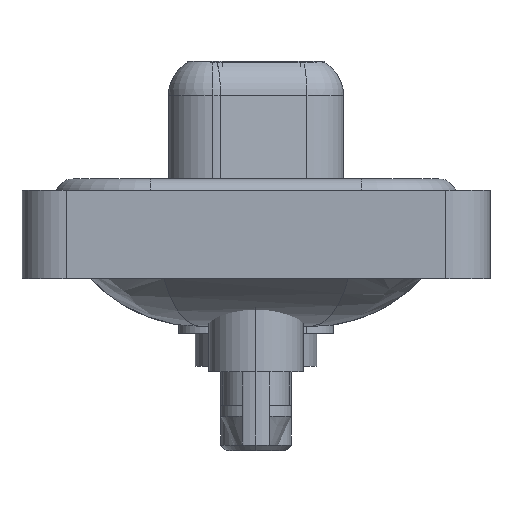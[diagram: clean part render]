
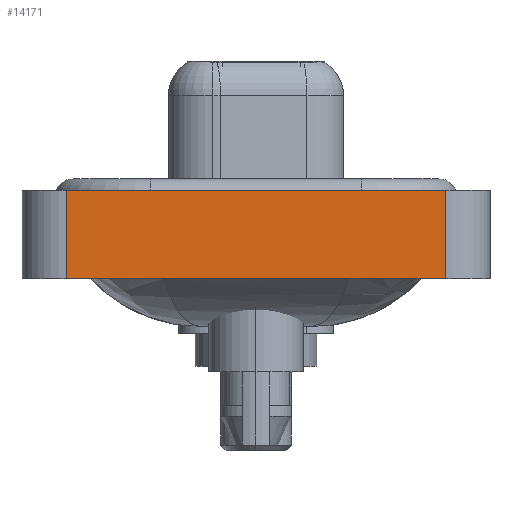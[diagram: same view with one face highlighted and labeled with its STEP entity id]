
A CAD part, left-side view. The second image highlights one B-rep face of the part: STEP entity #14171.
In plain terms, the highlighted planar face has unit normal (-1, 0, 0).
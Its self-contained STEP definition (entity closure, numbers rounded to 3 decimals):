
#54 = CARTESIAN_POINT ( 'NONE',  ( -7.35, 8.55, -3.6 ) ) ;
#336 = CARTESIAN_POINT ( 'NONE',  ( -7.35, -8.55, 0.4 ) ) ;
#414 = ORIENTED_EDGE ( 'NONE', *, *, #5938, .F. ) ;
#1872 = LINE ( 'NONE', #336, #3348 ) ;
#3235 = ORIENTED_EDGE ( 'NONE', *, *, #7629, .T. ) ;
#3348 = VECTOR ( 'NONE', #11578, 1000. ) ;
#3481 = CARTESIAN_POINT ( 'NONE',  ( -7.35, 8.55, -3.6 ) ) ;
#4111 = VERTEX_POINT ( 'NONE', #5325 ) ;
#4157 = DIRECTION ( 'NONE',  ( 0., -1., 0. ) ) ;
#5106 = LINE ( 'NONE', #15061, #16711 ) ;
#5325 = CARTESIAN_POINT ( 'NONE',  ( -7.35, -8.55, -3.6 ) ) ;
#5615 = DIRECTION ( 'NONE',  ( 0., 0., 1. ) ) ;
#5856 = DIRECTION ( 'NONE',  ( -1., 0., 0. ) ) ;
#5938 = EDGE_CURVE ( 'NONE', #7835, #12504, #1872, .T. ) ;
#7031 = DIRECTION ( 'NONE',  ( 0., 0., 1. ) ) ;
#7075 = ORIENTED_EDGE ( 'NONE', *, *, #15923, .T. ) ;
#7629 = EDGE_CURVE ( 'NONE', #17577, #4111, #12488, .T. ) ;
#7835 = VERTEX_POINT ( 'NONE', #17811 ) ;
#7854 = LINE ( 'NONE', #54, #12434 ) ;
#8200 = CARTESIAN_POINT ( 'NONE',  ( -7.35, -8.55, -3.6 ) ) ;
#9582 = DIRECTION ( 'NONE',  ( 0., 0., 1. ) ) ;
#10999 = AXIS2_PLACEMENT_3D ( 'NONE', #15433, #5856, #7031 ) ;
#11513 = EDGE_LOOP ( 'NONE', ( #7075, #414, #12401, #3235 ) ) ;
#11578 = DIRECTION ( 'NONE',  ( 0., -1., 0. ) ) ;
#12401 = ORIENTED_EDGE ( 'NONE', *, *, #13115, .F. ) ;
#12434 = VECTOR ( 'NONE', #5615, 1000. ) ;
#12488 = LINE ( 'NONE', #8200, #16452 ) ;
#12504 = VERTEX_POINT ( 'NONE', #15994 ) ;
#12712 = PLANE ( 'NONE',  #10999 ) ;
#12805 = FACE_OUTER_BOUND ( 'NONE', #11513, .T. ) ;
#13115 = EDGE_CURVE ( 'NONE', #17577, #7835, #7854, .T. ) ;
#14171 = ADVANCED_FACE ( 'NONE', ( #12805 ), #12712, .T. ) ;
#15061 = CARTESIAN_POINT ( 'NONE',  ( -7.35, -8.55, -3.6 ) ) ;
#15433 = CARTESIAN_POINT ( 'NONE',  ( -7.35, -8.55, -3.6 ) ) ;
#15923 = EDGE_CURVE ( 'NONE', #4111, #12504, #5106, .T. ) ;
#15994 = CARTESIAN_POINT ( 'NONE',  ( -7.35, -8.55, 0.4 ) ) ;
#16452 = VECTOR ( 'NONE', #4157, 1000. ) ;
#16711 = VECTOR ( 'NONE', #9582, 1000. ) ;
#17577 = VERTEX_POINT ( 'NONE', #3481 ) ;
#17811 = CARTESIAN_POINT ( 'NONE',  ( -7.35, 8.55, 0.4 ) ) ;
